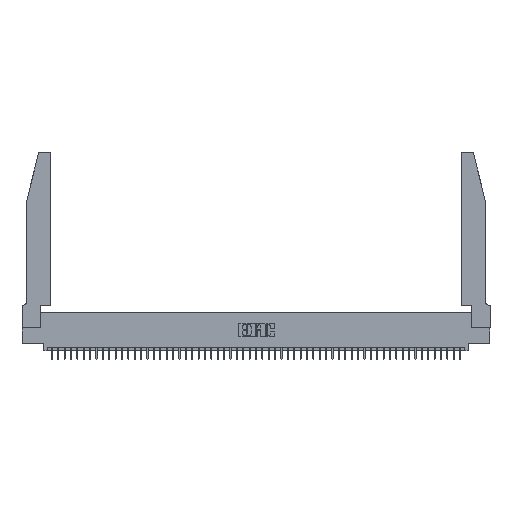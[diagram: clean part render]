
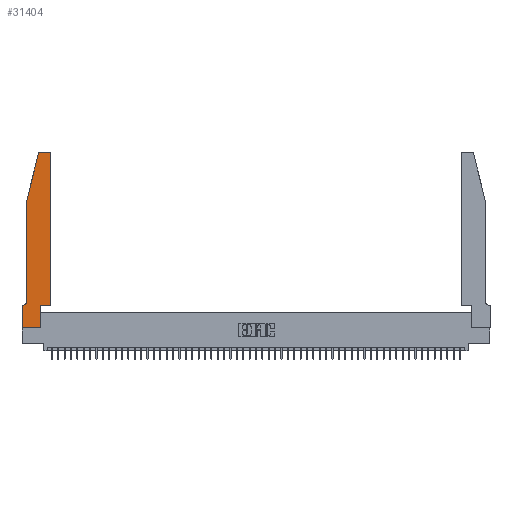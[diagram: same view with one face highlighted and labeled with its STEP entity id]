
A CAD part, top view. The second image highlights one B-rep face of the part: STEP entity #31404.
In plain terms, the highlighted planar face has unit normal (0, 0, 1).
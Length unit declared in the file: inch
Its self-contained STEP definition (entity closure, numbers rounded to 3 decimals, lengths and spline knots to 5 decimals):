
#562 = CARTESIAN_POINT ( 'NONE',  ( 0.0055, 0.42, 0.37 ) ) ;
#1766 = LINE ( 'NONE', #26118, #43126 ) ;
#2293 = VERTEX_POINT ( 'NONE', #31512 ) ;
#2605 = ORIENTED_EDGE ( 'NONE', *, *, #37055, .T. ) ;
#2615 = CARTESIAN_POINT ( 'NONE',  ( 0.4505, 0.35, 0.37 ) ) ;
#3520 = CARTESIAN_POINT ( 'NONE',  ( 0.0755, 2., 0.37 ) ) ;
#3900 = LINE ( 'NONE', #20194, #36573 ) ;
#4266 = VERTEX_POINT ( 'NONE', #9208 ) ;
#4957 = AXIS2_PLACEMENT_3D ( 'NONE', #51001, #26106, #25834 ) ;
#5377 = DIRECTION ( 'NONE',  ( -1., 0., 0. ) ) ;
#5831 = VERTEX_POINT ( 'NONE', #11369 ) ;
#5889 = DIRECTION ( 'NONE',  ( 0., 0., 1. ) ) ;
#5905 = CARTESIAN_POINT ( 'NONE',  ( 0., 0.35, 0.37 ) ) ;
#6242 = CARTESIAN_POINT ( 'NONE',  ( 0.2605, 2.75, 0.37 ) ) ;
#6265 = VECTOR ( 'NONE', #23034, 39.37008 ) ;
#6906 = CARTESIAN_POINT ( 'NONE',  ( 0.0755, 2., 0.37 ) ) ;
#7000 = ORIENTED_EDGE ( 'NONE', *, *, #20681, .T. ) ;
#7530 = LINE ( 'NONE', #3520, #6265 ) ;
#8696 = CARTESIAN_POINT ( 'NONE',  ( 0.0755, 2., 0.37 ) ) ;
#9151 = DIRECTION ( 'NONE',  ( 0., 1., 0. ) ) ;
#9208 = CARTESIAN_POINT ( 'NONE',  ( 0.284, 2.75, 0.37 ) ) ;
#9801 = VERTEX_POINT ( 'NONE', #38091 ) ;
#11369 = CARTESIAN_POINT ( 'NONE',  ( 0., 0., 0.37 ) ) ;
#11621 = CARTESIAN_POINT ( 'NONE',  ( 0.0755, 0.42, 0.37 ) ) ;
#13103 = DIRECTION ( 'NONE',  ( 0., 0., -1. ) ) ;
#13641 = AXIS2_PLACEMENT_3D ( 'NONE', #29460, #5889, #46848 ) ;
#14115 = LINE ( 'NONE', #6906, #43293 ) ;
#14161 = VERTEX_POINT ( 'NONE', #46872 ) ;
#14393 = DIRECTION ( 'NONE',  ( 0., -1., 0. ) ) ;
#14401 = ORIENTED_EDGE ( 'NONE', *, *, #35060, .T. ) ;
#14954 = EDGE_CURVE ( 'NONE', #4266, #31482, #28006, .T. ) ;
#15290 = ORIENTED_EDGE ( 'NONE', *, *, #16810, .T. ) ;
#15442 = VERTEX_POINT ( 'NONE', #47388 ) ;
#15713 = VECTOR ( 'NONE', #14393, 39.37008 ) ;
#16160 = DIRECTION ( 'NONE',  ( 1., 0., 0. ) ) ;
#16810 = EDGE_CURVE ( 'NONE', #14161, #4266, #34639, .T. ) ;
#17922 = CIRCLE ( 'NONE', #13641, 0.03 ) ;
#18049 = DIRECTION ( 'NONE',  ( 1., 0., 0. ) ) ;
#18199 = EDGE_CURVE ( 'NONE', #43947, #2293, #41303, .T. ) ;
#20083 = VERTEX_POINT ( 'NONE', #8696 ) ;
#20194 = CARTESIAN_POINT ( 'NONE',  ( 0.4505, 0.35, 0.37 ) ) ;
#20430 = EDGE_CURVE ( 'NONE', #31955, #15442, #36776, .T. ) ;
#20681 = EDGE_CURVE ( 'NONE', #20083, #27130, #7530, .T. ) ;
#21921 = ORIENTED_EDGE ( 'NONE', *, *, #20430, .T. ) ;
#23034 = DIRECTION ( 'NONE',  ( 0., -1., 0. ) ) ;
#23035 = VERTEX_POINT ( 'NONE', #36092 ) ;
#23110 = ORIENTED_EDGE ( 'NONE', *, *, #48669, .T. ) ;
#23744 = CARTESIAN_POINT ( 'NONE',  ( 0.2865, 0., 0.37 ) ) ;
#24091 = AXIS2_PLACEMENT_3D ( 'NONE', #562, #13103, #5377 ) ;
#25353 = ORIENTED_EDGE ( 'NONE', *, *, #18199, .T. ) ;
#25834 = DIRECTION ( 'NONE',  ( 1., 0., 0. ) ) ;
#26106 = DIRECTION ( 'NONE',  ( 0., 0., 1. ) ) ;
#26118 = CARTESIAN_POINT ( 'NONE',  ( 0., 0., 0.37 ) ) ;
#26159 = EDGE_LOOP ( 'NONE', ( #15290, #49679, #50995, #7000, #51327, #2605, #49154, #37016, #21921, #14401, #25353, #23110 ) ) ;
#27130 = VERTEX_POINT ( 'NONE', #11621 ) ;
#27284 = LINE ( 'NONE', #42839, #50754 ) ;
#28006 = CIRCLE ( 'NONE', #4957, 0.03 ) ;
#28703 = CARTESIAN_POINT ( 'NONE',  ( 0.2865, 0.35, 0.37 ) ) ;
#28974 = DIRECTION ( 'NONE',  ( 0., 1., 0. ) ) ;
#29460 = CARTESIAN_POINT ( 'NONE',  ( 0.4205, 2.72, 0.37 ) ) ;
#30593 = DIRECTION ( 'NONE',  ( -1., 0., 0. ) ) ;
#31321 = EDGE_CURVE ( 'NONE', #23035, #5831, #35583, .T. ) ;
#31322 = PLANE ( 'NONE',  #41469 ) ;
#31404 = ADVANCED_FACE ( 'NONE', ( #35347 ), #31322, .T. ) ;
#31482 = VERTEX_POINT ( 'NONE', #48183 ) ;
#31512 = CARTESIAN_POINT ( 'NONE',  ( 0.4505, 2.72, 0.37 ) ) ;
#31955 = VERTEX_POINT ( 'NONE', #23744 ) ;
#32084 = VECTOR ( 'NONE', #30593, 39.37008 ) ;
#33076 = EDGE_CURVE ( 'NONE', #31482, #20083, #14115, .T. ) ;
#34452 = VECTOR ( 'NONE', #28974, 39.37008 ) ;
#34639 = LINE ( 'NONE', #6242, #32084 ) ;
#35060 = EDGE_CURVE ( 'NONE', #15442, #43947, #3900, .T. ) ;
#35347 = FACE_OUTER_BOUND ( 'NONE', #26159, .T. ) ;
#35571 = DIRECTION ( 'NONE',  ( -0.239, -0.971, 0. ) ) ;
#35583 = LINE ( 'NONE', #47352, #15713 ) ;
#35611 = EDGE_CURVE ( 'NONE', #27130, #9801, #41252, .T. ) ;
#36092 = CARTESIAN_POINT ( 'NONE',  ( 0., 0.35, 0.37 ) ) ;
#36573 = VECTOR ( 'NONE', #16160, 39.37008 ) ;
#36776 = LINE ( 'NONE', #28703, #34452 ) ;
#37016 = ORIENTED_EDGE ( 'NONE', *, *, #37823, .T. ) ;
#37055 = EDGE_CURVE ( 'NONE', #9801, #23035, #27284, .T. ) ;
#37823 = EDGE_CURVE ( 'NONE', #5831, #31955, #1766, .T. ) ;
#38091 = CARTESIAN_POINT ( 'NONE',  ( 0.0055, 0.35, 0.37 ) ) ;
#38577 = DIRECTION ( 'NONE',  ( 1., 0., 0. ) ) ;
#41038 = CARTESIAN_POINT ( 'NONE',  ( 0.4505, 0.35, 0.37 ) ) ;
#41252 = CIRCLE ( 'NONE', #24091, 0.07 ) ;
#41303 = LINE ( 'NONE', #41038, #48936 ) ;
#41469 = AXIS2_PLACEMENT_3D ( 'NONE', #5905, #42591, #38577 ) ;
#42591 = DIRECTION ( 'NONE',  ( 0., 0., 1. ) ) ;
#42839 = CARTESIAN_POINT ( 'NONE',  ( 0.0755, 0.35, 0.37 ) ) ;
#43126 = VECTOR ( 'NONE', #18049, 39.37008 ) ;
#43293 = VECTOR ( 'NONE', #35571, 39.37008 ) ;
#43947 = VERTEX_POINT ( 'NONE', #2615 ) ;
#46848 = DIRECTION ( 'NONE',  ( 1., 0., 0. ) ) ;
#46872 = CARTESIAN_POINT ( 'NONE',  ( 0.4205, 2.75, 0.37 ) ) ;
#47113 = DIRECTION ( 'NONE',  ( -1., 0., 0. ) ) ;
#47352 = CARTESIAN_POINT ( 'NONE',  ( 0., 0., 0.37 ) ) ;
#47388 = CARTESIAN_POINT ( 'NONE',  ( 0.2865, 0.35, 0.37 ) ) ;
#48183 = CARTESIAN_POINT ( 'NONE',  ( 0.25487, 2.72718, 0.37 ) ) ;
#48669 = EDGE_CURVE ( 'NONE', #2293, #14161, #17922, .T. ) ;
#48936 = VECTOR ( 'NONE', #9151, 39.37008 ) ;
#49154 = ORIENTED_EDGE ( 'NONE', *, *, #31321, .T. ) ;
#49679 = ORIENTED_EDGE ( 'NONE', *, *, #14954, .T. ) ;
#50754 = VECTOR ( 'NONE', #47113, 39.37008 ) ;
#50995 = ORIENTED_EDGE ( 'NONE', *, *, #33076, .T. ) ;
#51001 = CARTESIAN_POINT ( 'NONE',  ( 0.284, 2.72, 0.37 ) ) ;
#51327 = ORIENTED_EDGE ( 'NONE', *, *, #35611, .T. ) ;
